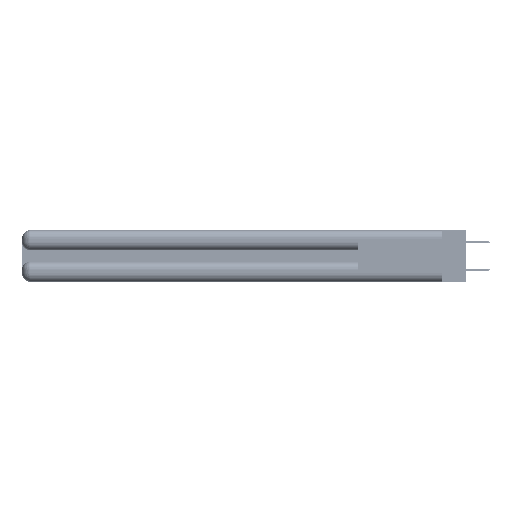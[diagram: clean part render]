
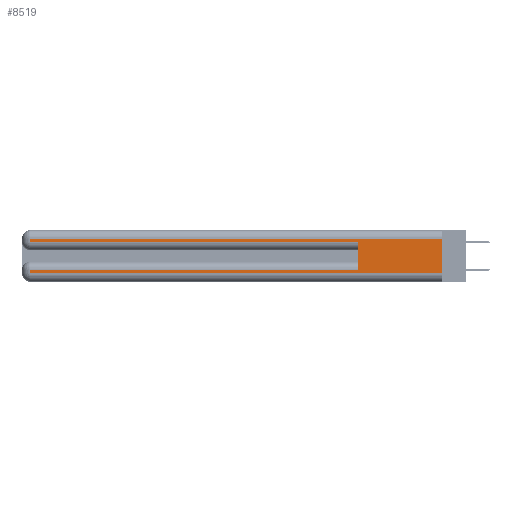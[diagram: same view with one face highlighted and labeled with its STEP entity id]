
A CAD part, left-side view. The second image highlights one B-rep face of the part: STEP entity #8519.
In plain terms, the highlighted planar face has unit normal (-1, 0, 0).
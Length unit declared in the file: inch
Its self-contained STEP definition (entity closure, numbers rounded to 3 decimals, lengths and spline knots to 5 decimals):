
#1310 = CARTESIAN_POINT ( 'NONE',  ( 0., 0.6, 0.285 ) ) ;
#1376 = VERTEX_POINT ( 'NONE', #50106 ) ;
#1832 = ORIENTED_EDGE ( 'NONE', *, *, #27978, .T. ) ;
#1911 = VERTEX_POINT ( 'NONE', #10457 ) ;
#4523 = ORIENTED_EDGE ( 'NONE', *, *, #21346, .F. ) ;
#5172 = CARTESIAN_POINT ( 'NONE',  ( 0., 0., 0.37 ) ) ;
#5363 = ORIENTED_EDGE ( 'NONE', *, *, #53930, .T. ) ;
#5897 = CARTESIAN_POINT ( 'NONE',  ( 0., 0., 0.37 ) ) ;
#6070 = LINE ( 'NONE', #43678, #29626 ) ;
#6114 = LINE ( 'NONE', #5897, #38637 ) ;
#6236 = CARTESIAN_POINT ( 'NONE',  ( 0., 2.94, 0.06 ) ) ;
#8519 = ADVANCED_FACE ( 'NONE', ( #35641 ), #40545, .F. ) ;
#8927 = CARTESIAN_POINT ( 'NONE',  ( 0., 0., 0.06 ) ) ;
#9032 = LINE ( 'NONE', #50565, #53258 ) ;
#10457 = CARTESIAN_POINT ( 'NONE',  ( 0., 2.94, 0.31 ) ) ;
#10790 = LINE ( 'NONE', #13860, #43229 ) ;
#13860 = CARTESIAN_POINT ( 'NONE',  ( 0., 0., 0.06 ) ) ;
#14123 = DIRECTION ( 'NONE',  ( 1., 0., 0. ) ) ;
#16677 = CARTESIAN_POINT ( 'NONE',  ( 0., 2.94, 0.37 ) ) ;
#17246 = DIRECTION ( 'NONE',  ( 0., -1., 0. ) ) ;
#17296 = DIRECTION ( 'NONE',  ( 0., 1., 0. ) ) ;
#18271 = LINE ( 'NONE', #16677, #40325 ) ;
#19306 = CARTESIAN_POINT ( 'NONE',  ( 0., 0.6, 0.145 ) ) ;
#20543 = LINE ( 'NONE', #30412, #54315 ) ;
#21137 = DIRECTION ( 'NONE',  ( 0., 0., -1. ) ) ;
#21346 = EDGE_CURVE ( 'NONE', #52051, #36746, #6114, .T. ) ;
#21465 = CARTESIAN_POINT ( 'NONE',  ( 0., 2.94, 0.085 ) ) ;
#23272 = EDGE_CURVE ( 'NONE', #42163, #36746, #10790, .T. ) ;
#23393 = EDGE_CURVE ( 'NONE', #41085, #49647, #48040, .T. ) ;
#23527 = CARTESIAN_POINT ( 'NONE',  ( 0., 0., 0.085 ) ) ;
#23759 = DIRECTION ( 'NONE',  ( 0., 0., 1. ) ) ;
#24597 = VECTOR ( 'NONE', #37046, 39.37008 ) ;
#27175 = DIRECTION ( 'NONE',  ( 0., -1., 0. ) ) ;
#27978 = EDGE_CURVE ( 'NONE', #1911, #1376, #9032, .T. ) ;
#28555 = DIRECTION ( 'NONE',  ( 0., 0., -1. ) ) ;
#29626 = VECTOR ( 'NONE', #17246, 39.37008 ) ;
#29717 = EDGE_CURVE ( 'NONE', #41085, #55925, #37290, .T. ) ;
#30412 = CARTESIAN_POINT ( 'NONE',  ( 0., 0., 0.31 ) ) ;
#35641 = FACE_OUTER_BOUND ( 'NONE', #40664, .T. ) ;
#36746 = VERTEX_POINT ( 'NONE', #8927 ) ;
#36871 = DIRECTION ( 'NONE',  ( 0., 0., -1. ) ) ;
#37046 = DIRECTION ( 'NONE',  ( 0., 1., 0. ) ) ;
#37290 = LINE ( 'NONE', #19306, #38648 ) ;
#38004 = CARTESIAN_POINT ( 'NONE',  ( 0., 0., 0.31 ) ) ;
#38379 = ORIENTED_EDGE ( 'NONE', *, *, #23393, .T. ) ;
#38524 = AXIS2_PLACEMENT_3D ( 'NONE', #5172, #14123, #44999 ) ;
#38637 = VECTOR ( 'NONE', #36871, 39.37008 ) ;
#38648 = VECTOR ( 'NONE', #23759, 39.37008 ) ;
#40325 = VECTOR ( 'NONE', #21137, 39.37008 ) ;
#40545 = PLANE ( 'NONE',  #38524 ) ;
#40664 = EDGE_LOOP ( 'NONE', ( #4523, #5363, #1832, #42894, #44223, #38379, #55451, #40977 ) ) ;
#40977 = ORIENTED_EDGE ( 'NONE', *, *, #23272, .T. ) ;
#41085 = VERTEX_POINT ( 'NONE', #55225 ) ;
#42163 = VERTEX_POINT ( 'NONE', #6236 ) ;
#42894 = ORIENTED_EDGE ( 'NONE', *, *, #52569, .T. ) ;
#43229 = VECTOR ( 'NONE', #27175, 39.37008 ) ;
#43678 = CARTESIAN_POINT ( 'NONE',  ( 0., 0., 0.285 ) ) ;
#44223 = ORIENTED_EDGE ( 'NONE', *, *, #29717, .F. ) ;
#44714 = EDGE_CURVE ( 'NONE', #49647, #42163, #18271, .T. ) ;
#44999 = DIRECTION ( 'NONE',  ( 0., 0., -1. ) ) ;
#48040 = LINE ( 'NONE', #23527, #24597 ) ;
#49647 = VERTEX_POINT ( 'NONE', #21465 ) ;
#50106 = CARTESIAN_POINT ( 'NONE',  ( 0., 2.94, 0.285 ) ) ;
#50565 = CARTESIAN_POINT ( 'NONE',  ( 0., 2.94, 0.37 ) ) ;
#52051 = VERTEX_POINT ( 'NONE', #38004 ) ;
#52569 = EDGE_CURVE ( 'NONE', #1376, #55925, #6070, .T. ) ;
#53258 = VECTOR ( 'NONE', #28555, 39.37008 ) ;
#53930 = EDGE_CURVE ( 'NONE', #52051, #1911, #20543, .T. ) ;
#54315 = VECTOR ( 'NONE', #17296, 39.37008 ) ;
#55225 = CARTESIAN_POINT ( 'NONE',  ( 0., 0.6, 0.085 ) ) ;
#55451 = ORIENTED_EDGE ( 'NONE', *, *, #44714, .T. ) ;
#55925 = VERTEX_POINT ( 'NONE', #1310 ) ;
